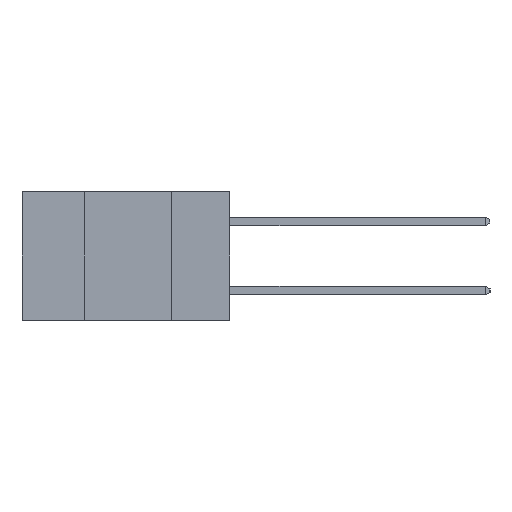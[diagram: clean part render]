
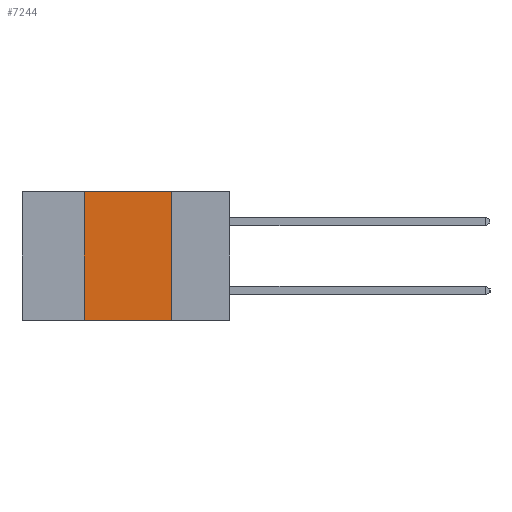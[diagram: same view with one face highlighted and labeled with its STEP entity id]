
A CAD part, left-side view. The second image highlights one B-rep face of the part: STEP entity #7244.
In plain terms, the highlighted planar face has unit normal (-1, 0, 0).
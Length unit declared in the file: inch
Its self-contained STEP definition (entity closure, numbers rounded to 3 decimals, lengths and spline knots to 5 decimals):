
#118 = FACE_OUTER_BOUND ( 'NONE', #11724, .T. ) ;
#189 = VERTEX_POINT ( 'NONE', #13973 ) ;
#471 = EDGE_CURVE ( 'NONE', #12788, #12439, #10753, .T. ) ;
#1374 = VECTOR ( 'NONE', #18913, 39.37008 ) ;
#1656 = VECTOR ( 'NONE', #16342, 39.37008 ) ;
#2217 = CARTESIAN_POINT ( 'NONE',  ( 0., 0.17, 0. ) ) ;
#2300 = LINE ( 'NONE', #2366, #13369 ) ;
#2366 = CARTESIAN_POINT ( 'NONE',  ( 0., 0.42, -0.37 ) ) ;
#2890 = DIRECTION ( 'NONE',  ( 1., 0., 0. ) ) ;
#4194 = EDGE_CURVE ( 'NONE', #12439, #189, #19592, .T. ) ;
#5151 = ORIENTED_EDGE ( 'NONE', *, *, #4194, .F. ) ;
#5916 = CARTESIAN_POINT ( 'NONE',  ( 0., 0.6, 0. ) ) ;
#6064 = DIRECTION ( 'NONE',  ( 0., 0., 1. ) ) ;
#6638 = CARTESIAN_POINT ( 'NONE',  ( 0., 0.42, 0. ) ) ;
#7244 = ADVANCED_FACE ( 'NONE', ( #118 ), #9901, .F. ) ;
#7348 = VECTOR ( 'NONE', #8423, 39.37008 ) ;
#7924 = VERTEX_POINT ( 'NONE', #8222 ) ;
#8222 = CARTESIAN_POINT ( 'NONE',  ( 0., 0.42, -0.37 ) ) ;
#8423 = DIRECTION ( 'NONE',  ( 0., -1., 0. ) ) ;
#9901 = PLANE ( 'NONE',  #15436 ) ;
#9946 = ORIENTED_EDGE ( 'NONE', *, *, #16949, .T. ) ;
#10753 = LINE ( 'NONE', #5916, #1374 ) ;
#11724 = EDGE_LOOP ( 'NONE', ( #5151, #13773, #14306, #9946 ) ) ;
#12439 = VERTEX_POINT ( 'NONE', #2217 ) ;
#12741 = LINE ( 'NONE', #13286, #7348 ) ;
#12788 = VERTEX_POINT ( 'NONE', #6638 ) ;
#13165 = CARTESIAN_POINT ( 'NONE',  ( 0., 0.6, 0. ) ) ;
#13286 = CARTESIAN_POINT ( 'NONE',  ( 0., 0.6, -0.37 ) ) ;
#13369 = VECTOR ( 'NONE', #6064, 39.37008 ) ;
#13773 = ORIENTED_EDGE ( 'NONE', *, *, #471, .F. ) ;
#13973 = CARTESIAN_POINT ( 'NONE',  ( 0., 0.17, -0.37 ) ) ;
#14306 = ORIENTED_EDGE ( 'NONE', *, *, #21271, .F. ) ;
#14790 = DIRECTION ( 'NONE',  ( 0., 0., -1. ) ) ;
#15436 = AXIS2_PLACEMENT_3D ( 'NONE', #13165, #2890, #14790 ) ;
#16074 = CARTESIAN_POINT ( 'NONE',  ( 0., 0.17, -0.37 ) ) ;
#16342 = DIRECTION ( 'NONE',  ( 0., 0., -1. ) ) ;
#16949 = EDGE_CURVE ( 'NONE', #7924, #189, #12741, .T. ) ;
#18913 = DIRECTION ( 'NONE',  ( 0., -1., 0. ) ) ;
#19592 = LINE ( 'NONE', #16074, #1656 ) ;
#21271 = EDGE_CURVE ( 'NONE', #7924, #12788, #2300, .T. ) ;
